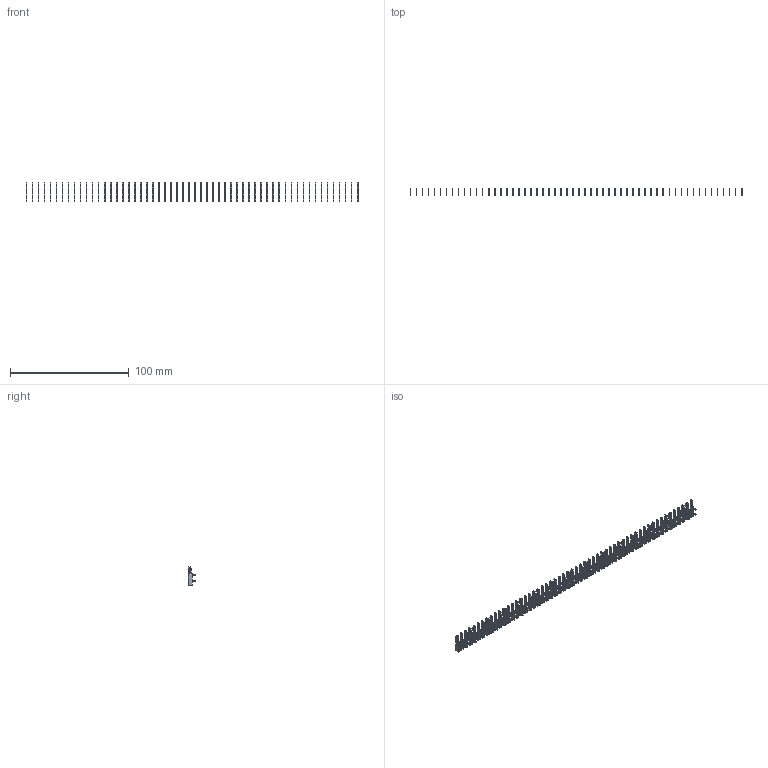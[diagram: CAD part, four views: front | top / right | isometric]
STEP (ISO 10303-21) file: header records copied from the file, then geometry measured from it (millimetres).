
FILE_DESCRIPTION (( 'STEP AP203' ), '1' );
FILE_NAME ('105-056-202-200.STEP', '2020-04-08T00:43:32', ( '' ), ( '' ), 'SwSTEP 2.0', 'SolidWorks 2016', '' );
FILE_SCHEMA (( 'CONFIG_CONTROL_DESIGN' ));
Length unit declared in the file: inch
Products named in the file (2): 105-056-202-200; 100-290-001_100-290-202
Assembly tree (56 placements, depth 2):
  105-056-202-200
    100-290-001_100-290-202  x56
Bounding box: 280 x 6.53 x 15.88 mm (x, y, z)
Volume: 1779.2 mm3; surface area: 7912.8 mm2
Topology: 56 solids, 56 shells, 1680 faces, 4704 edges, 3136 vertices
Faces by surface type: plane 1288, cylinder 392
Entity records: 2922 total; most frequent: DIRECTION 272, CARTESIAN_POINT 241, ORIENTED_EDGE 168, CALENDAR_DATE 122, DATE_AND_TIME 122, COORDINATED_UNIVERSAL_TIME_OFFSET 122, LOCAL_TIME 122, AXIS2_PLACEMENT_3D 103
